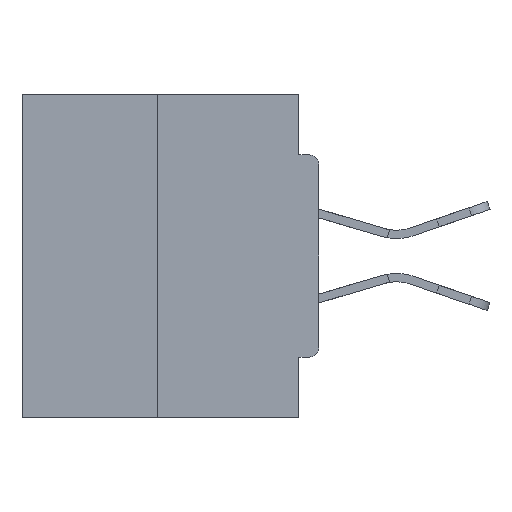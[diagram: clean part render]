
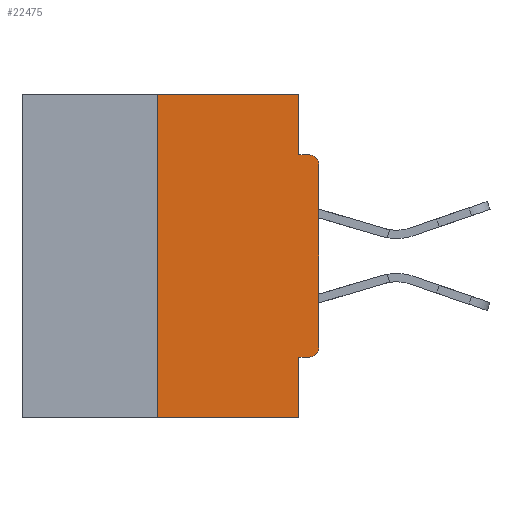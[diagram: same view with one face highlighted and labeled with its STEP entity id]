
A CAD part, left-side view. The second image highlights one B-rep face of the part: STEP entity #22475.
In plain terms, the highlighted planar face has unit normal (-1, 0, 0).
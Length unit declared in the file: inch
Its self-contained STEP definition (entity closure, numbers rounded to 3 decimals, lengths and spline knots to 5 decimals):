
#304 = DIRECTION ( 'NONE',  ( 0., 0., -1. ) ) ;
#1172 = CARTESIAN_POINT ( 'NONE',  ( 0., 0.46, -0.5 ) ) ;
#1256 = CARTESIAN_POINT ( 'NONE',  ( 0., 0., -0.1085 ) ) ;
#1814 = CARTESIAN_POINT ( 'NONE',  ( 0., 0.031, -0.4065 ) ) ;
#1998 = AXIS2_PLACEMENT_3D ( 'NONE', #18600, #27812, #23221 ) ;
#2921 = EDGE_CURVE ( 'NONE', #28263, #12951, #34148, .T. ) ;
#3358 = VERTEX_POINT ( 'NONE', #3551 ) ;
#3405 = CARTESIAN_POINT ( 'NONE',  ( 0., 0.031, -0.5 ) ) ;
#3551 = CARTESIAN_POINT ( 'NONE',  ( 0., 0.015, -0.4065 ) ) ;
#3782 = VERTEX_POINT ( 'NONE', #5532 ) ;
#3931 = ORIENTED_EDGE ( 'NONE', *, *, #35125, .F. ) ;
#3956 = ORIENTED_EDGE ( 'NONE', *, *, #10352, .F. ) ;
#4031 = FACE_OUTER_BOUND ( 'NONE', #10592, .T. ) ;
#4058 = VECTOR ( 'NONE', #25003, 39.37008 ) ;
#4273 = ORIENTED_EDGE ( 'NONE', *, *, #6547, .T. ) ;
#4924 = DIRECTION ( 'NONE',  ( 0., 0., 1. ) ) ;
#5509 = VECTOR ( 'NONE', #14766, 39.37008 ) ;
#5532 = CARTESIAN_POINT ( 'NONE',  ( 0., 0.031, -0.0935 ) ) ;
#5786 = VECTOR ( 'NONE', #4924, 39.37008 ) ;
#5936 = EDGE_CURVE ( 'NONE', #3358, #11985, #24112, .T. ) ;
#6020 = CARTESIAN_POINT ( 'NONE',  ( 0., 0.46, 0. ) ) ;
#6271 = DIRECTION ( 'NONE',  ( 0., -1., 0. ) ) ;
#6547 = EDGE_CURVE ( 'NONE', #16336, #30983, #19161, .T. ) ;
#8242 = AXIS2_PLACEMENT_3D ( 'NONE', #28596, #28710, #304 ) ;
#8412 = AXIS2_PLACEMENT_3D ( 'NONE', #31097, #22239, #10792 ) ;
#8498 = VERTEX_POINT ( 'NONE', #1814 ) ;
#9369 = EDGE_CURVE ( 'NONE', #3782, #30983, #30577, .T. ) ;
#9385 = CARTESIAN_POINT ( 'NONE',  ( 0., 0.031, -0.5 ) ) ;
#9984 = VERTEX_POINT ( 'NONE', #34619 ) ;
#10022 = EDGE_CURVE ( 'NONE', #3358, #8498, #15345, .T. ) ;
#10352 = EDGE_CURVE ( 'NONE', #9984, #3782, #18015, .T. ) ;
#10592 = EDGE_LOOP ( 'NONE', ( #29321, #3931, #36122, #18424, #14363, #25777, #12604, #4273, #20039, #3956 ) ) ;
#10792 = DIRECTION ( 'NONE',  ( 0., 0., -1. ) ) ;
#10970 = CARTESIAN_POINT ( 'NONE',  ( 0., 0.25, 0. ) ) ;
#11985 = VERTEX_POINT ( 'NONE', #30199 ) ;
#12135 = LINE ( 'NONE', #13664, #4058 ) ;
#12604 = ORIENTED_EDGE ( 'NONE', *, *, #29008, .T. ) ;
#12951 = VERTEX_POINT ( 'NONE', #3405 ) ;
#13385 = EDGE_CURVE ( 'NONE', #36790, #9984, #32972, .T. ) ;
#13664 = CARTESIAN_POINT ( 'NONE',  ( 0., 0.25, 0. ) ) ;
#14248 = LINE ( 'NONE', #24642, #5786 ) ;
#14363 = ORIENTED_EDGE ( 'NONE', *, *, #10022, .F. ) ;
#14766 = DIRECTION ( 'NONE',  ( 0., 1., 0. ) ) ;
#15345 = LINE ( 'NONE', #32125, #5509 ) ;
#15834 = VECTOR ( 'NONE', #32221, 39.37008 ) ;
#16202 = DIRECTION ( 'NONE',  ( 0., 0., -1. ) ) ;
#16336 = VERTEX_POINT ( 'NONE', #1256 ) ;
#17696 = LINE ( 'NONE', #9385, #34229 ) ;
#17761 = EDGE_CURVE ( 'NONE', #8498, #12951, #17696, .T. ) ;
#18015 = LINE ( 'NONE', #30456, #26021 ) ;
#18424 = ORIENTED_EDGE ( 'NONE', *, *, #17761, .F. ) ;
#18600 = CARTESIAN_POINT ( 'NONE',  ( 0., 0.015, -0.1085 ) ) ;
#19161 = CIRCLE ( 'NONE', #1998, 0.015 ) ;
#19234 = CARTESIAN_POINT ( 'NONE',  ( 0., 0.25, -0.5 ) ) ;
#20039 = ORIENTED_EDGE ( 'NONE', *, *, #9369, .F. ) ;
#22239 = DIRECTION ( 'NONE',  ( 1., 0., 0. ) ) ;
#22475 = ADVANCED_FACE ( 'NONE', ( #4031 ), #25355, .F. ) ;
#23221 = DIRECTION ( 'NONE',  ( 0., 0., -1. ) ) ;
#24112 = CIRCLE ( 'NONE', #8242, 0.015 ) ;
#24642 = CARTESIAN_POINT ( 'NONE',  ( 0., 0., 0. ) ) ;
#24766 = VECTOR ( 'NONE', #26193, 39.37008 ) ;
#25003 = DIRECTION ( 'NONE',  ( 0., 0., 1. ) ) ;
#25355 = PLANE ( 'NONE',  #8412 ) ;
#25777 = ORIENTED_EDGE ( 'NONE', *, *, #5936, .T. ) ;
#26021 = VECTOR ( 'NONE', #16202, 39.37008 ) ;
#26193 = DIRECTION ( 'NONE',  ( 0., -1., 0. ) ) ;
#27812 = DIRECTION ( 'NONE',  ( -1., 0., 0. ) ) ;
#28091 = VECTOR ( 'NONE', #6271, 39.37008 ) ;
#28263 = VERTEX_POINT ( 'NONE', #19234 ) ;
#28596 = CARTESIAN_POINT ( 'NONE',  ( 0., 0.015, -0.3915 ) ) ;
#28710 = DIRECTION ( 'NONE',  ( -1., 0., 0. ) ) ;
#29008 = EDGE_CURVE ( 'NONE', #11985, #16336, #14248, .T. ) ;
#29321 = ORIENTED_EDGE ( 'NONE', *, *, #13385, .F. ) ;
#29327 = DIRECTION ( 'NONE',  ( 0., 0., -1. ) ) ;
#30199 = CARTESIAN_POINT ( 'NONE',  ( 0., 0., -0.3915 ) ) ;
#30456 = CARTESIAN_POINT ( 'NONE',  ( 0., 0.031, 0. ) ) ;
#30577 = LINE ( 'NONE', #34541, #24766 ) ;
#30983 = VERTEX_POINT ( 'NONE', #32167 ) ;
#31097 = CARTESIAN_POINT ( 'NONE',  ( 0., 0.46, 0. ) ) ;
#32125 = CARTESIAN_POINT ( 'NONE',  ( 0., 0., -0.4065 ) ) ;
#32167 = CARTESIAN_POINT ( 'NONE',  ( 0., 0.015, -0.0935 ) ) ;
#32221 = DIRECTION ( 'NONE',  ( 0., -1., 0. ) ) ;
#32972 = LINE ( 'NONE', #6020, #28091 ) ;
#34148 = LINE ( 'NONE', #1172, #15834 ) ;
#34229 = VECTOR ( 'NONE', #29327, 39.37008 ) ;
#34541 = CARTESIAN_POINT ( 'NONE',  ( 0., 0., -0.0935 ) ) ;
#34619 = CARTESIAN_POINT ( 'NONE',  ( 0., 0.031, 0. ) ) ;
#35125 = EDGE_CURVE ( 'NONE', #28263, #36790, #12135, .T. ) ;
#36122 = ORIENTED_EDGE ( 'NONE', *, *, #2921, .T. ) ;
#36790 = VERTEX_POINT ( 'NONE', #10970 ) ;
